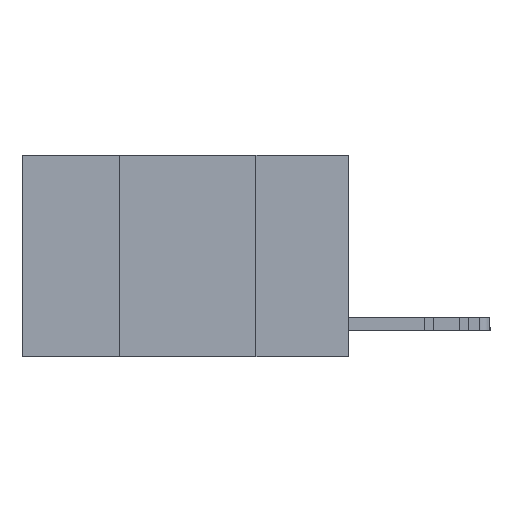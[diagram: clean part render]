
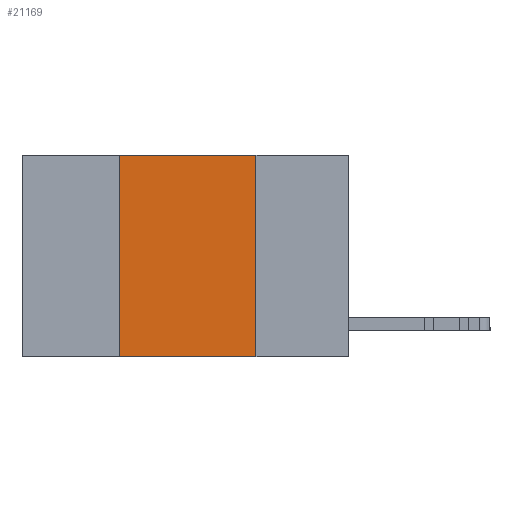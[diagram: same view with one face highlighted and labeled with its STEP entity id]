
A CAD part, left-side view. The second image highlights one B-rep face of the part: STEP entity #21169.
In plain terms, the highlighted planar face has unit normal (-1, 0, 0).
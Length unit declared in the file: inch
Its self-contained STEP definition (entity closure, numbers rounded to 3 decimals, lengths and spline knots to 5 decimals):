
#1679 = DIRECTION ( 'NONE',  ( 0., 0., -1. ) ) ;
#2764 = ORIENTED_EDGE ( 'NONE', *, *, #12836, .T. ) ;
#4029 = PLANE ( 'NONE',  #26119 ) ;
#4628 = CARTESIAN_POINT ( 'NONE',  ( 0., 0.6, 0. ) ) ;
#4654 = CARTESIAN_POINT ( 'NONE',  ( 0., 0.17, -0.37 ) ) ;
#6439 = ORIENTED_EDGE ( 'NONE', *, *, #25018, .F. ) ;
#6731 = LINE ( 'NONE', #9057, #9944 ) ;
#7460 = VERTEX_POINT ( 'NONE', #28884 ) ;
#7593 = LINE ( 'NONE', #14737, #19673 ) ;
#8833 = FACE_OUTER_BOUND ( 'NONE', #30173, .T. ) ;
#9057 = CARTESIAN_POINT ( 'NONE',  ( 0., 0.42, 0. ) ) ;
#9944 = VECTOR ( 'NONE', #16189, 39.37008 ) ;
#10739 = CARTESIAN_POINT ( 'NONE',  ( 0., 0.17, 0. ) ) ;
#12836 = EDGE_CURVE ( 'NONE', #13293, #19448, #17959, .T. ) ;
#13293 = VERTEX_POINT ( 'NONE', #29867 ) ;
#13299 = LINE ( 'NONE', #25279, #17863 ) ;
#14225 = VERTEX_POINT ( 'NONE', #10739 ) ;
#14737 = CARTESIAN_POINT ( 'NONE',  ( 0., 0.6, 0. ) ) ;
#15841 = VECTOR ( 'NONE', #27446, 39.37008 ) ;
#16189 = DIRECTION ( 'NONE',  ( 0., 0., 1. ) ) ;
#17863 = VECTOR ( 'NONE', #20278, 39.37008 ) ;
#17959 = LINE ( 'NONE', #20430, #15841 ) ;
#19245 = ORIENTED_EDGE ( 'NONE', *, *, #25546, .F. ) ;
#19448 = VERTEX_POINT ( 'NONE', #4654 ) ;
#19673 = VECTOR ( 'NONE', #24232, 39.37008 ) ;
#20278 = DIRECTION ( 'NONE',  ( 0., 0., -1. ) ) ;
#20430 = CARTESIAN_POINT ( 'NONE',  ( 0., 0.6, -0.37 ) ) ;
#20907 = EDGE_CURVE ( 'NONE', #7460, #14225, #7593, .T. ) ;
#20930 = DIRECTION ( 'NONE',  ( 1., 0., 0. ) ) ;
#21169 = ADVANCED_FACE ( 'NONE', ( #8833 ), #4029, .F. ) ;
#23397 = ORIENTED_EDGE ( 'NONE', *, *, #20907, .F. ) ;
#24232 = DIRECTION ( 'NONE',  ( 0., -1., 0. ) ) ;
#25018 = EDGE_CURVE ( 'NONE', #14225, #19448, #13299, .T. ) ;
#25279 = CARTESIAN_POINT ( 'NONE',  ( 0., 0.17, 0. ) ) ;
#25546 = EDGE_CURVE ( 'NONE', #13293, #7460, #6731, .T. ) ;
#26119 = AXIS2_PLACEMENT_3D ( 'NONE', #4628, #20930, #1679 ) ;
#27446 = DIRECTION ( 'NONE',  ( 0., -1., 0. ) ) ;
#28884 = CARTESIAN_POINT ( 'NONE',  ( 0., 0.42, 0. ) ) ;
#29867 = CARTESIAN_POINT ( 'NONE',  ( 0., 0.42, -0.37 ) ) ;
#30173 = EDGE_LOOP ( 'NONE', ( #6439, #23397, #19245, #2764 ) ) ;
